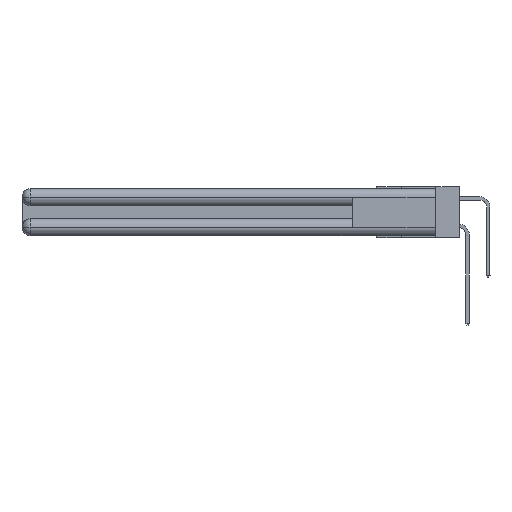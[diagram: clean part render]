
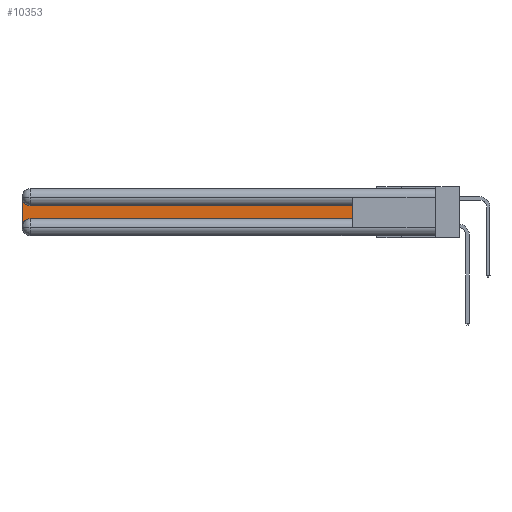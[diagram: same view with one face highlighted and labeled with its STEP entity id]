
A CAD part, left-side view. The second image highlights one B-rep face of the part: STEP entity #10353.
In plain terms, the highlighted planar face has unit normal (-1, 0, 0).
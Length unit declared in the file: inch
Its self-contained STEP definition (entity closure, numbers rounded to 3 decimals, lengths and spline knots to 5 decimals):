
#155 = CIRCLE ( 'NONE', #4765, 0.06 ) ;
#714 = EDGE_CURVE ( 'NONE', #9731, #30760, #28246, .T. ) ;
#1636 = LINE ( 'NONE', #27219, #26759 ) ;
#1919 = FACE_OUTER_BOUND ( 'NONE', #17410, .T. ) ;
#2123 = VERTEX_POINT ( 'NONE', #19186 ) ;
#2193 = PLANE ( 'NONE',  #16167 ) ;
#3030 = DIRECTION ( 'NONE',  ( 1., 0., 0. ) ) ;
#4045 = DIRECTION ( 'NONE',  ( 0., -1., 0. ) ) ;
#4066 = CARTESIAN_POINT ( 'NONE',  ( 0.075, 0.6, -0.1225 ) ) ;
#4191 = CIRCLE ( 'NONE', #8633, 0.06 ) ;
#4765 = AXIS2_PLACEMENT_3D ( 'NONE', #14005, #16773, #30917 ) ;
#5663 = ORIENTED_EDGE ( 'NONE', *, *, #28065, .T. ) ;
#5751 = EDGE_CURVE ( 'NONE', #20769, #12083, #13979, .T. ) ;
#7318 = CARTESIAN_POINT ( 'NONE',  ( 0.075, 3., -0.0625 ) ) ;
#7735 = CARTESIAN_POINT ( 'NONE',  ( 0.075, 3., -0.1225 ) ) ;
#8633 = AXIS2_PLACEMENT_3D ( 'NONE', #13950, #3030, #22395 ) ;
#8640 = ORIENTED_EDGE ( 'NONE', *, *, #714, .T. ) ;
#9731 = VERTEX_POINT ( 'NONE', #7318 ) ;
#10353 = ADVANCED_FACE ( 'NONE', ( #1919 ), #2193, .F. ) ;
#11800 = VECTOR ( 'NONE', #16007, 39.37008 ) ;
#12083 = VERTEX_POINT ( 'NONE', #4066 ) ;
#13533 = CARTESIAN_POINT ( 'NONE',  ( 0.075, 2.94, -0.2175 ) ) ;
#13950 = CARTESIAN_POINT ( 'NONE',  ( 0.075, 2.94, -0.2775 ) ) ;
#13979 = LINE ( 'NONE', #31508, #11800 ) ;
#14005 = CARTESIAN_POINT ( 'NONE',  ( 0.075, 2.94, -0.0625 ) ) ;
#16007 = DIRECTION ( 'NONE',  ( 0., 0., 1. ) ) ;
#16167 = AXIS2_PLACEMENT_3D ( 'NONE', #7735, #32795, #35583 ) ;
#16773 = DIRECTION ( 'NONE',  ( 1., 0., 0. ) ) ;
#17410 = EDGE_LOOP ( 'NONE', ( #28358, #5663, #8640, #25164, #29607, #21838 ) ) ;
#19186 = CARTESIAN_POINT ( 'NONE',  ( 0.075, 2.94, -0.1225 ) ) ;
#20769 = VERTEX_POINT ( 'NONE', #27210 ) ;
#20853 = CARTESIAN_POINT ( 'NONE',  ( 0.075, 3., -0.2175 ) ) ;
#21838 = ORIENTED_EDGE ( 'NONE', *, *, #5751, .T. ) ;
#22035 = EDGE_CURVE ( 'NONE', #34769, #20769, #30076, .T. ) ;
#22239 = CARTESIAN_POINT ( 'NONE',  ( 0.075, 3., -0.2775 ) ) ;
#22395 = DIRECTION ( 'NONE',  ( 0., 0., -1. ) ) ;
#23738 = DIRECTION ( 'NONE',  ( 0., 0., -1. ) ) ;
#24042 = VECTOR ( 'NONE', #4045, 39.37008 ) ;
#25164 = ORIENTED_EDGE ( 'NONE', *, *, #35754, .T. ) ;
#25780 = EDGE_CURVE ( 'NONE', #12083, #2123, #1636, .T. ) ;
#26759 = VECTOR ( 'NONE', #35564, 39.37008 ) ;
#26953 = VECTOR ( 'NONE', #23738, 39.37008 ) ;
#27210 = CARTESIAN_POINT ( 'NONE',  ( 0.075, 0.6, -0.2175 ) ) ;
#27219 = CARTESIAN_POINT ( 'NONE',  ( 0.075, 0.6, -0.1225 ) ) ;
#28065 = EDGE_CURVE ( 'NONE', #2123, #9731, #155, .T. ) ;
#28246 = LINE ( 'NONE', #20853, #26953 ) ;
#28358 = ORIENTED_EDGE ( 'NONE', *, *, #25780, .T. ) ;
#29607 = ORIENTED_EDGE ( 'NONE', *, *, #22035, .T. ) ;
#30076 = LINE ( 'NONE', #34296, #24042 ) ;
#30760 = VERTEX_POINT ( 'NONE', #22239 ) ;
#30917 = DIRECTION ( 'NONE',  ( 0., 0., -1. ) ) ;
#31508 = CARTESIAN_POINT ( 'NONE',  ( 0.075, 0.6, -0.2175 ) ) ;
#32795 = DIRECTION ( 'NONE',  ( 1., 0., 0. ) ) ;
#34296 = CARTESIAN_POINT ( 'NONE',  ( 0.075, 0.6, -0.2175 ) ) ;
#34769 = VERTEX_POINT ( 'NONE', #13533 ) ;
#35564 = DIRECTION ( 'NONE',  ( 0., 1., 0. ) ) ;
#35583 = DIRECTION ( 'NONE',  ( 0., 0., -1. ) ) ;
#35754 = EDGE_CURVE ( 'NONE', #30760, #34769, #4191, .T. ) ;
